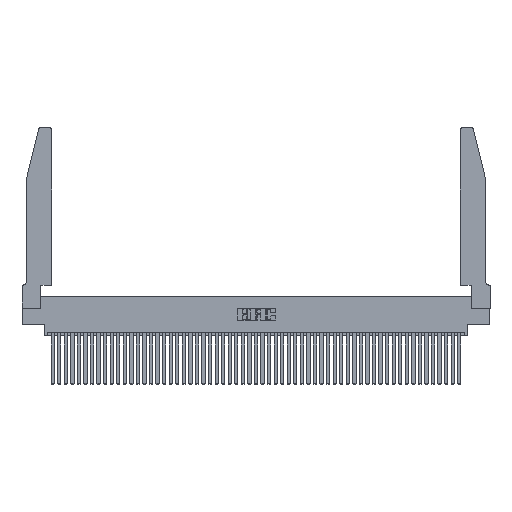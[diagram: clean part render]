
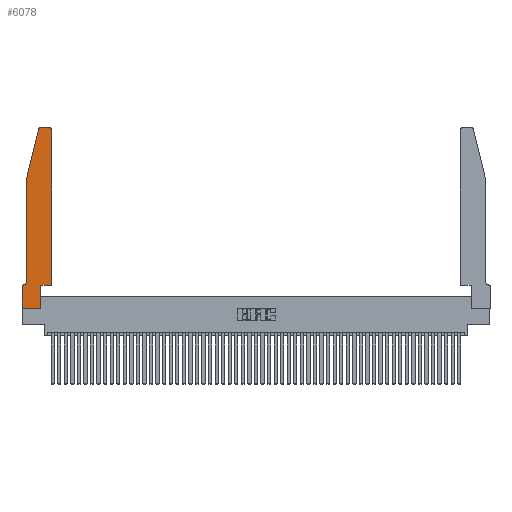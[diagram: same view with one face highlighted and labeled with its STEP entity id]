
A CAD part, top view. The second image highlights one B-rep face of the part: STEP entity #6078.
In plain terms, the highlighted planar face has unit normal (0, 0, 1).
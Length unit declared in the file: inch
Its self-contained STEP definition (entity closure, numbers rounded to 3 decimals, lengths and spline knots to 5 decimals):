
#56 = VECTOR ( 'NONE', #41973, 39.37008 ) ;
#202 = CARTESIAN_POINT ( 'NONE',  ( 0.0055, 0.42, 0.37 ) ) ;
#1139 = CARTESIAN_POINT ( 'NONE',  ( 0., 0., 0.37 ) ) ;
#1313 = CARTESIAN_POINT ( 'NONE',  ( 0.2605, 2.75, 0.37 ) ) ;
#1476 = CARTESIAN_POINT ( 'NONE',  ( 0.0755, 0.42, 0.37 ) ) ;
#2270 = ORIENTED_EDGE ( 'NONE', *, *, #10625, .T. ) ;
#2443 = VERTEX_POINT ( 'NONE', #26377 ) ;
#2531 = EDGE_CURVE ( 'NONE', #49405, #12112, #2638, .T. ) ;
#2638 = CIRCLE ( 'NONE', #27784, 0.03 ) ;
#2689 = ORIENTED_EDGE ( 'NONE', *, *, #43890, .T. ) ;
#3261 = PLANE ( 'NONE',  #12557 ) ;
#3604 = ORIENTED_EDGE ( 'NONE', *, *, #38239, .T. ) ;
#3722 = LINE ( 'NONE', #50196, #36613 ) ;
#4085 = LINE ( 'NONE', #46098, #44977 ) ;
#4291 = DIRECTION ( 'NONE',  ( -1., 0., 0. ) ) ;
#4502 = CARTESIAN_POINT ( 'NONE',  ( 0.25487, 2.72718, 0.37 ) ) ;
#5411 = DIRECTION ( 'NONE',  ( -1., 0., 0. ) ) ;
#6078 = ADVANCED_FACE ( 'NONE', ( #28484 ), #3261, .T. ) ;
#6477 = VERTEX_POINT ( 'NONE', #13277 ) ;
#6884 = AXIS2_PLACEMENT_3D ( 'NONE', #202, #28182, #4291 ) ;
#7318 = DIRECTION ( 'NONE',  ( 1., 0., 0. ) ) ;
#7791 = CARTESIAN_POINT ( 'NONE',  ( 0.284, 2.72, 0.37 ) ) ;
#7994 = CARTESIAN_POINT ( 'NONE',  ( 0.0755, 0.35, 0.37 ) ) ;
#10625 = EDGE_CURVE ( 'NONE', #40983, #51283, #3722, .T. ) ;
#10649 = CARTESIAN_POINT ( 'NONE',  ( 0.284, 2.75, 0.37 ) ) ;
#10895 = CARTESIAN_POINT ( 'NONE',  ( 0.4205, 2.72, 0.37 ) ) ;
#11214 = VERTEX_POINT ( 'NONE', #10649 ) ;
#11805 = DIRECTION ( 'NONE',  ( 1., 0., 0. ) ) ;
#12017 = CARTESIAN_POINT ( 'NONE',  ( 0.0755, 2., 0.37 ) ) ;
#12112 = VERTEX_POINT ( 'NONE', #28619 ) ;
#12557 = AXIS2_PLACEMENT_3D ( 'NONE', #50664, #19242, #7318 ) ;
#13036 = CARTESIAN_POINT ( 'NONE',  ( 0., 0., 0.37 ) ) ;
#13273 = LINE ( 'NONE', #1313, #34243 ) ;
#13277 = CARTESIAN_POINT ( 'NONE',  ( 0., 0.35, 0.37 ) ) ;
#13549 = CARTESIAN_POINT ( 'NONE',  ( 0.4505, 2.72, 0.37 ) ) ;
#13869 = EDGE_CURVE ( 'NONE', #35447, #49405, #4085, .T. ) ;
#14933 = CARTESIAN_POINT ( 'NONE',  ( 0.2865, 0.35, 0.37 ) ) ;
#14940 = DIRECTION ( 'NONE',  ( 1., 0., 0. ) ) ;
#15505 = ORIENTED_EDGE ( 'NONE', *, *, #21982, .T. ) ;
#16924 = ORIENTED_EDGE ( 'NONE', *, *, #20877, .T. ) ;
#16997 = VECTOR ( 'NONE', #21728, 39.37008 ) ;
#17232 = LINE ( 'NONE', #43301, #26531 ) ;
#18088 = LINE ( 'NONE', #1139, #48216 ) ;
#19242 = DIRECTION ( 'NONE',  ( 0., 0., 1. ) ) ;
#19610 = EDGE_CURVE ( 'NONE', #2443, #24883, #17232, .T. ) ;
#19933 = VERTEX_POINT ( 'NONE', #1476 ) ;
#20081 = LINE ( 'NONE', #7994, #50155 ) ;
#20111 = DIRECTION ( 'NONE',  ( -1., 0., 0. ) ) ;
#20229 = LINE ( 'NONE', #38026, #56 ) ;
#20877 = EDGE_CURVE ( 'NONE', #11214, #40983, #25629, .T. ) ;
#21728 = DIRECTION ( 'NONE',  ( 0., -1., 0. ) ) ;
#21982 = EDGE_CURVE ( 'NONE', #6477, #47794, #18088, .T. ) ;
#22181 = CARTESIAN_POINT ( 'NONE',  ( 0., 0., 0.37 ) ) ;
#23783 = DIRECTION ( 'NONE',  ( 0., 1., 0. ) ) ;
#24883 = VERTEX_POINT ( 'NONE', #14933 ) ;
#25307 = ORIENTED_EDGE ( 'NONE', *, *, #42523, .T. ) ;
#25629 = CIRCLE ( 'NONE', #33825, 0.03 ) ;
#26377 = CARTESIAN_POINT ( 'NONE',  ( 0.2865, 0., 0.37 ) ) ;
#26531 = VECTOR ( 'NONE', #23783, 39.37008 ) ;
#27010 = EDGE_CURVE ( 'NONE', #51283, #19933, #37905, .T. ) ;
#27318 = LINE ( 'NONE', #22181, #37697 ) ;
#27784 = AXIS2_PLACEMENT_3D ( 'NONE', #10895, #38516, #14940 ) ;
#28182 = DIRECTION ( 'NONE',  ( 0., 0., -1. ) ) ;
#28484 = FACE_OUTER_BOUND ( 'NONE', #50166, .T. ) ;
#28619 = CARTESIAN_POINT ( 'NONE',  ( 0.4205, 2.75, 0.37 ) ) ;
#28906 = ORIENTED_EDGE ( 'NONE', *, *, #47355, .T. ) ;
#30054 = DIRECTION ( 'NONE',  ( 1., 0., 0. ) ) ;
#33825 = AXIS2_PLACEMENT_3D ( 'NONE', #7791, #35465, #11805 ) ;
#33835 = ORIENTED_EDGE ( 'NONE', *, *, #37760, .T. ) ;
#34243 = VECTOR ( 'NONE', #5411, 39.37008 ) ;
#34647 = ORIENTED_EDGE ( 'NONE', *, *, #13869, .T. ) ;
#34722 = CARTESIAN_POINT ( 'NONE',  ( 0.0055, 0.35, 0.37 ) ) ;
#35447 = VERTEX_POINT ( 'NONE', #43943 ) ;
#35465 = DIRECTION ( 'NONE',  ( 0., 0., 1. ) ) ;
#36613 = VECTOR ( 'NONE', #46235, 39.37008 ) ;
#37697 = VECTOR ( 'NONE', #30054, 39.37008 ) ;
#37760 = EDGE_CURVE ( 'NONE', #12112, #11214, #13273, .T. ) ;
#37905 = LINE ( 'NONE', #41227, #16997 ) ;
#38026 = CARTESIAN_POINT ( 'NONE',  ( 0.4505, 0.35, 0.37 ) ) ;
#38239 = EDGE_CURVE ( 'NONE', #19933, #44979, #47100, .T. ) ;
#38516 = DIRECTION ( 'NONE',  ( 0., 0., 1. ) ) ;
#40983 = VERTEX_POINT ( 'NONE', #4502 ) ;
#41227 = CARTESIAN_POINT ( 'NONE',  ( 0.0755, 2., 0.37 ) ) ;
#41973 = DIRECTION ( 'NONE',  ( 1., 0., 0. ) ) ;
#42523 = EDGE_CURVE ( 'NONE', #24883, #35447, #20229, .T. ) ;
#43301 = CARTESIAN_POINT ( 'NONE',  ( 0.2865, 0.35, 0.37 ) ) ;
#43890 = EDGE_CURVE ( 'NONE', #44979, #6477, #20081, .T. ) ;
#43943 = CARTESIAN_POINT ( 'NONE',  ( 0.4505, 0.35, 0.37 ) ) ;
#44671 = ORIENTED_EDGE ( 'NONE', *, *, #19610, .T. ) ;
#44847 = DIRECTION ( 'NONE',  ( 0., -1., 0. ) ) ;
#44977 = VECTOR ( 'NONE', #50065, 39.37008 ) ;
#44979 = VERTEX_POINT ( 'NONE', #34722 ) ;
#46098 = CARTESIAN_POINT ( 'NONE',  ( 0.4505, 0.35, 0.37 ) ) ;
#46235 = DIRECTION ( 'NONE',  ( -0.239, -0.971, 0. ) ) ;
#46654 = ORIENTED_EDGE ( 'NONE', *, *, #2531, .T. ) ;
#47100 = CIRCLE ( 'NONE', #6884, 0.07 ) ;
#47355 = EDGE_CURVE ( 'NONE', #47794, #2443, #27318, .T. ) ;
#47794 = VERTEX_POINT ( 'NONE', #13036 ) ;
#48216 = VECTOR ( 'NONE', #44847, 39.37008 ) ;
#48937 = ORIENTED_EDGE ( 'NONE', *, *, #27010, .T. ) ;
#49405 = VERTEX_POINT ( 'NONE', #13549 ) ;
#50065 = DIRECTION ( 'NONE',  ( 0., 1., 0. ) ) ;
#50155 = VECTOR ( 'NONE', #20111, 39.37008 ) ;
#50166 = EDGE_LOOP ( 'NONE', ( #33835, #16924, #2270, #48937, #3604, #2689, #15505, #28906, #44671, #25307, #34647, #46654 ) ) ;
#50196 = CARTESIAN_POINT ( 'NONE',  ( 0.0755, 2., 0.37 ) ) ;
#50664 = CARTESIAN_POINT ( 'NONE',  ( 0., 0.35, 0.37 ) ) ;
#51283 = VERTEX_POINT ( 'NONE', #12017 ) ;
